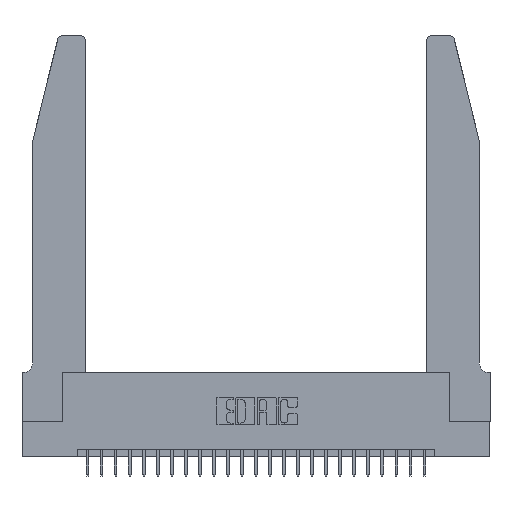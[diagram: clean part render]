
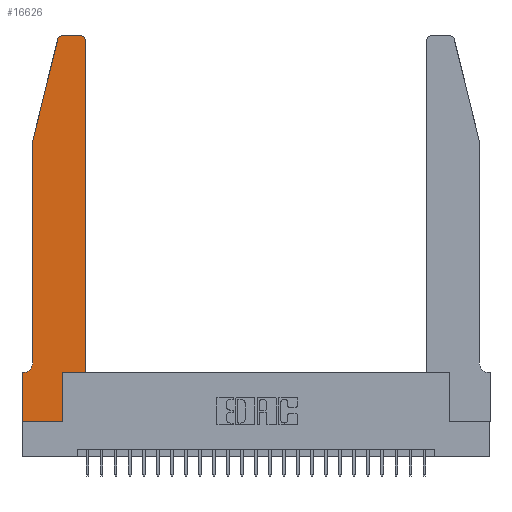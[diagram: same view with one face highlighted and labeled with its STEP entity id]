
A CAD part, top view. The second image highlights one B-rep face of the part: STEP entity #16626.
In plain terms, the highlighted planar face has unit normal (0, 0, 1).
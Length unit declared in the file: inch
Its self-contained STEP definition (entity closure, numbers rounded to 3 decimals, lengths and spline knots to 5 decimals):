
#1 = CARTESIAN_POINT ( 'NONE',  ( 0.284, 2.72, 0.37 ) ) ;
#77 = VERTEX_POINT ( 'NONE', #4907 ) ;
#185 = EDGE_CURVE ( 'NONE', #77, #24713, #9656, .T. ) ;
#612 = CARTESIAN_POINT ( 'NONE',  ( 0.4505, 2.72, 0.37 ) ) ;
#1030 = CARTESIAN_POINT ( 'NONE',  ( 0.2865, 0.35, 0.37 ) ) ;
#1060 = DIRECTION ( 'NONE',  ( 0., -1., 0. ) ) ;
#1146 = VECTOR ( 'NONE', #18404, 39.37008 ) ;
#1645 = CIRCLE ( 'NONE', #24175, 0.03 ) ;
#1816 = CARTESIAN_POINT ( 'NONE',  ( 0.2865, 0.35, 0.37 ) ) ;
#1964 = DIRECTION ( 'NONE',  ( 0., 0., 1. ) ) ;
#2065 = CARTESIAN_POINT ( 'NONE',  ( 0.0755, 2., 0.37 ) ) ;
#2365 = DIRECTION ( 'NONE',  ( 0., 0., -1. ) ) ;
#3214 = CARTESIAN_POINT ( 'NONE',  ( 0., 0., 0.37 ) ) ;
#3406 = CARTESIAN_POINT ( 'NONE',  ( 0., 0.35, 0.37 ) ) ;
#3621 = VERTEX_POINT ( 'NONE', #26341 ) ;
#3904 = VECTOR ( 'NONE', #7303, 39.37008 ) ;
#4326 = ORIENTED_EDGE ( 'NONE', *, *, #16779, .T. ) ;
#4604 = DIRECTION ( 'NONE',  ( -0.239, -0.971, 0. ) ) ;
#4767 = DIRECTION ( 'NONE',  ( 1., 0., 0. ) ) ;
#4907 = CARTESIAN_POINT ( 'NONE',  ( 0.4505, 0.35, 0.37 ) ) ;
#4996 = CIRCLE ( 'NONE', #21963, 0.07 ) ;
#5366 = CARTESIAN_POINT ( 'NONE',  ( 0., 0., 0.37 ) ) ;
#5409 = EDGE_CURVE ( 'NONE', #16907, #20451, #11005, .T. ) ;
#5659 = VERTEX_POINT ( 'NONE', #11077 ) ;
#5856 = PLANE ( 'NONE',  #11020 ) ;
#6774 = ORIENTED_EDGE ( 'NONE', *, *, #17916, .T. ) ;
#6848 = VERTEX_POINT ( 'NONE', #14540 ) ;
#7085 = EDGE_CURVE ( 'NONE', #19090, #18365, #21875, .T. ) ;
#7087 = EDGE_CURVE ( 'NONE', #5659, #16907, #4996, .T. ) ;
#7303 = DIRECTION ( 'NONE',  ( -1., 0., 0. ) ) ;
#7752 = EDGE_CURVE ( 'NONE', #18365, #11470, #26678, .T. ) ;
#8226 = DIRECTION ( 'NONE',  ( 0., 1., 0. ) ) ;
#8294 = DIRECTION ( 'NONE',  ( -1., 0., 0. ) ) ;
#9249 = AXIS2_PLACEMENT_3D ( 'NONE', #25396, #15127, #4767 ) ;
#9383 = ORIENTED_EDGE ( 'NONE', *, *, #7087, .T. ) ;
#9512 = ORIENTED_EDGE ( 'NONE', *, *, #21168, .T. ) ;
#9656 = LINE ( 'NONE', #24343, #1146 ) ;
#10017 = DIRECTION ( 'NONE',  ( 1., 0., 0. ) ) ;
#10313 = VERTEX_POINT ( 'NONE', #24292 ) ;
#10463 = DIRECTION ( 'NONE',  ( 0., -1., 0. ) ) ;
#10515 = ORIENTED_EDGE ( 'NONE', *, *, #7085, .T. ) ;
#10869 = LINE ( 'NONE', #22717, #13927 ) ;
#10871 = EDGE_CURVE ( 'NONE', #6848, #5659, #10869, .T. ) ;
#11005 = LINE ( 'NONE', #15347, #3904 ) ;
#11020 = AXIS2_PLACEMENT_3D ( 'NONE', #14191, #1964, #22639 ) ;
#11077 = CARTESIAN_POINT ( 'NONE',  ( 0.0755, 0.42, 0.37 ) ) ;
#11470 = VERTEX_POINT ( 'NONE', #1030 ) ;
#11523 = DIRECTION ( 'NONE',  ( 1., 0., 0. ) ) ;
#11826 = ORIENTED_EDGE ( 'NONE', *, *, #23579, .T. ) ;
#12002 = EDGE_LOOP ( 'NONE', ( #16882, #11826, #17924, #14102, #9383, #26512, #9512, #10515, #20164, #6774, #14838, #4326 ) ) ;
#12184 = CARTESIAN_POINT ( 'NONE',  ( 0., 0., 0.37 ) ) ;
#12795 = VECTOR ( 'NONE', #25281, 39.37008 ) ;
#13927 = VECTOR ( 'NONE', #10463, 39.37008 ) ;
#14102 = ORIENTED_EDGE ( 'NONE', *, *, #10871, .T. ) ;
#14191 = CARTESIAN_POINT ( 'NONE',  ( 0., 0.35, 0.37 ) ) ;
#14540 = CARTESIAN_POINT ( 'NONE',  ( 0.0755, 2., 0.37 ) ) ;
#14703 = EDGE_CURVE ( 'NONE', #10313, #3621, #24721, .T. ) ;
#14838 = ORIENTED_EDGE ( 'NONE', *, *, #185, .T. ) ;
#15127 = DIRECTION ( 'NONE',  ( 0., 0., 1. ) ) ;
#15347 = CARTESIAN_POINT ( 'NONE',  ( 0.0755, 0.35, 0.37 ) ) ;
#15594 = LINE ( 'NONE', #5366, #25058 ) ;
#15844 = DIRECTION ( 'NONE',  ( 0., 0., 1. ) ) ;
#15907 = CARTESIAN_POINT ( 'NONE',  ( 0.0055, 0.35, 0.37 ) ) ;
#16243 = FACE_OUTER_BOUND ( 'NONE', #12002, .T. ) ;
#16626 = ADVANCED_FACE ( 'NONE', ( #16243 ), #5856, .T. ) ;
#16779 = EDGE_CURVE ( 'NONE', #24713, #10313, #26162, .T. ) ;
#16794 = CARTESIAN_POINT ( 'NONE',  ( 0.4505, 0.35, 0.37 ) ) ;
#16882 = ORIENTED_EDGE ( 'NONE', *, *, #14703, .T. ) ;
#16907 = VERTEX_POINT ( 'NONE', #15907 ) ;
#17010 = EDGE_CURVE ( 'NONE', #20417, #6848, #20696, .T. ) ;
#17916 = EDGE_CURVE ( 'NONE', #11470, #77, #23035, .T. ) ;
#17924 = ORIENTED_EDGE ( 'NONE', *, *, #17010, .T. ) ;
#18365 = VERTEX_POINT ( 'NONE', #23510 ) ;
#18404 = DIRECTION ( 'NONE',  ( 0., 1., 0. ) ) ;
#18673 = CARTESIAN_POINT ( 'NONE',  ( 0.2605, 2.75, 0.37 ) ) ;
#19090 = VERTEX_POINT ( 'NONE', #12184 ) ;
#19837 = CARTESIAN_POINT ( 'NONE',  ( 0.0055, 0.42, 0.37 ) ) ;
#20164 = ORIENTED_EDGE ( 'NONE', *, *, #7752, .T. ) ;
#20417 = VERTEX_POINT ( 'NONE', #26308 ) ;
#20451 = VERTEX_POINT ( 'NONE', #3406 ) ;
#20696 = LINE ( 'NONE', #2065, #24044 ) ;
#21168 = EDGE_CURVE ( 'NONE', #20451, #19090, #15594, .T. ) ;
#21875 = LINE ( 'NONE', #3214, #25791 ) ;
#21963 = AXIS2_PLACEMENT_3D ( 'NONE', #19837, #2365, #25152 ) ;
#22434 = VECTOR ( 'NONE', #8226, 39.37008 ) ;
#22639 = DIRECTION ( 'NONE',  ( 1., 0., 0. ) ) ;
#22717 = CARTESIAN_POINT ( 'NONE',  ( 0.0755, 2., 0.37 ) ) ;
#23035 = LINE ( 'NONE', #16794, #12795 ) ;
#23510 = CARTESIAN_POINT ( 'NONE',  ( 0.2865, 0., 0.37 ) ) ;
#23579 = EDGE_CURVE ( 'NONE', #3621, #20417, #1645, .T. ) ;
#24044 = VECTOR ( 'NONE', #4604, 39.37008 ) ;
#24175 = AXIS2_PLACEMENT_3D ( 'NONE', #1, #15844, #10017 ) ;
#24292 = CARTESIAN_POINT ( 'NONE',  ( 0.4205, 2.75, 0.37 ) ) ;
#24343 = CARTESIAN_POINT ( 'NONE',  ( 0.4505, 0.35, 0.37 ) ) ;
#24470 = VECTOR ( 'NONE', #8294, 39.37008 ) ;
#24713 = VERTEX_POINT ( 'NONE', #612 ) ;
#24721 = LINE ( 'NONE', #18673, #24470 ) ;
#25058 = VECTOR ( 'NONE', #1060, 39.37008 ) ;
#25152 = DIRECTION ( 'NONE',  ( -1., 0., 0. ) ) ;
#25281 = DIRECTION ( 'NONE',  ( 1., 0., 0. ) ) ;
#25396 = CARTESIAN_POINT ( 'NONE',  ( 0.4205, 2.72, 0.37 ) ) ;
#25791 = VECTOR ( 'NONE', #11523, 39.37008 ) ;
#26162 = CIRCLE ( 'NONE', #9249, 0.03 ) ;
#26308 = CARTESIAN_POINT ( 'NONE',  ( 0.25487, 2.72718, 0.37 ) ) ;
#26341 = CARTESIAN_POINT ( 'NONE',  ( 0.284, 2.75, 0.37 ) ) ;
#26512 = ORIENTED_EDGE ( 'NONE', *, *, #5409, .T. ) ;
#26678 = LINE ( 'NONE', #1816, #22434 ) ;
